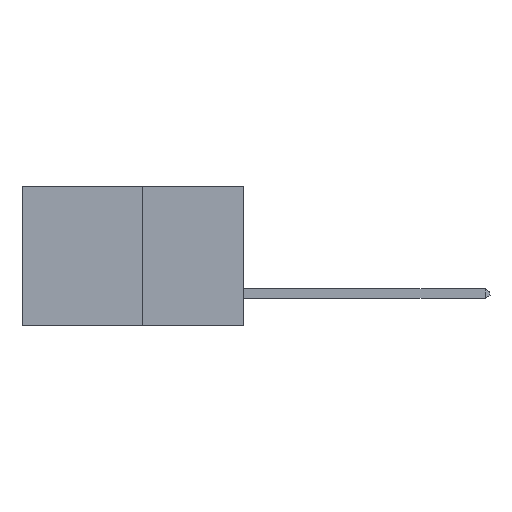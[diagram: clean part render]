
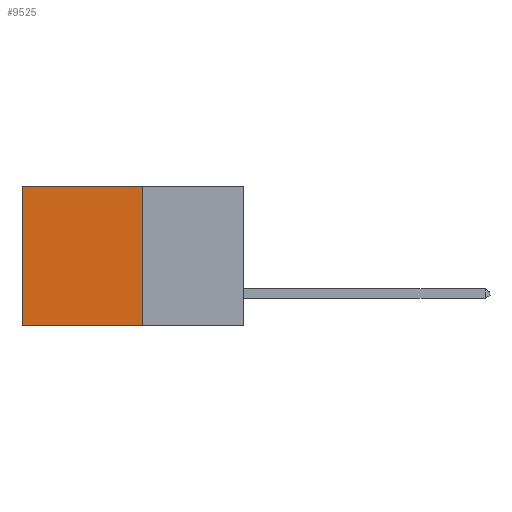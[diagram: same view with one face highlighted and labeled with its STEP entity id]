
A CAD part, left-side view. The second image highlights one B-rep face of the part: STEP entity #9525.
In plain terms, the highlighted planar face has unit normal (-1, 0, 0).
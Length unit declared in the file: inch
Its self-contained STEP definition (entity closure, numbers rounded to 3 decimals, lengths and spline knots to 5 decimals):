
#310 = CARTESIAN_POINT ( 'NONE',  ( 0.277, 0.27, -0.37 ) ) ;
#354 = VERTEX_POINT ( 'NONE', #8133 ) ;
#595 = CARTESIAN_POINT ( 'NONE',  ( 0.277, 0.27, -0.37 ) ) ;
#637 = PLANE ( 'NONE',  #7338 ) ;
#1095 = DIRECTION ( 'NONE',  ( 0., 1., 0. ) ) ;
#1611 = DIRECTION ( 'NONE',  ( 0., 0., -1. ) ) ;
#1690 = DIRECTION ( 'NONE',  ( 0., 0., -1. ) ) ;
#1835 = LINE ( 'NONE', #2637, #11354 ) ;
#2637 = CARTESIAN_POINT ( 'NONE',  ( 0.277, 0.27, 0. ) ) ;
#3228 = VECTOR ( 'NONE', #11520, 39.37008 ) ;
#3915 = VECTOR ( 'NONE', #1611, 39.37008 ) ;
#4248 = EDGE_CURVE ( 'NONE', #6039, #6148, #1835, .T. ) ;
#4488 = ORIENTED_EDGE ( 'NONE', *, *, #7458, .T. ) ;
#4499 = ORIENTED_EDGE ( 'NONE', *, *, #10398, .F. ) ;
#4602 = ORIENTED_EDGE ( 'NONE', *, *, #8037, .F. ) ;
#4625 = ORIENTED_EDGE ( 'NONE', *, *, #4248, .T. ) ;
#4709 = FACE_OUTER_BOUND ( 'NONE', #11676, .T. ) ;
#5377 = VERTEX_POINT ( 'NONE', #11802 ) ;
#5834 = LINE ( 'NONE', #310, #3228 ) ;
#6039 = VERTEX_POINT ( 'NONE', #9742 ) ;
#6148 = VERTEX_POINT ( 'NONE', #8415 ) ;
#6405 = VECTOR ( 'NONE', #9254, 39.37008 ) ;
#6619 = CARTESIAN_POINT ( 'NONE',  ( 0.277, 0.27, -0.37 ) ) ;
#7338 = AXIS2_PLACEMENT_3D ( 'NONE', #6619, #7509, #1690 ) ;
#7458 = EDGE_CURVE ( 'NONE', #6148, #354, #10792, .T. ) ;
#7509 = DIRECTION ( 'NONE',  ( 1., 0., 0. ) ) ;
#8037 = EDGE_CURVE ( 'NONE', #6039, #5377, #5834, .T. ) ;
#8133 = CARTESIAN_POINT ( 'NONE',  ( 0.277, 0.59, -0.37 ) ) ;
#8415 = CARTESIAN_POINT ( 'NONE',  ( 0.277, 0.59, 0. ) ) ;
#8769 = LINE ( 'NONE', #595, #6405 ) ;
#9254 = DIRECTION ( 'NONE',  ( 0., 1., 0. ) ) ;
#9525 = ADVANCED_FACE ( 'NONE', ( #4709 ), #637, .F. ) ;
#9742 = CARTESIAN_POINT ( 'NONE',  ( 0.277, 0.27, 0. ) ) ;
#10398 = EDGE_CURVE ( 'NONE', #5377, #354, #8769, .T. ) ;
#10792 = LINE ( 'NONE', #11737, #3915 ) ;
#11354 = VECTOR ( 'NONE', #1095, 39.37008 ) ;
#11520 = DIRECTION ( 'NONE',  ( 0., 0., -1. ) ) ;
#11676 = EDGE_LOOP ( 'NONE', ( #4488, #4499, #4602, #4625 ) ) ;
#11737 = CARTESIAN_POINT ( 'NONE',  ( 0.277, 0.59, -0.37 ) ) ;
#11802 = CARTESIAN_POINT ( 'NONE',  ( 0.277, 0.27, -0.37 ) ) ;
